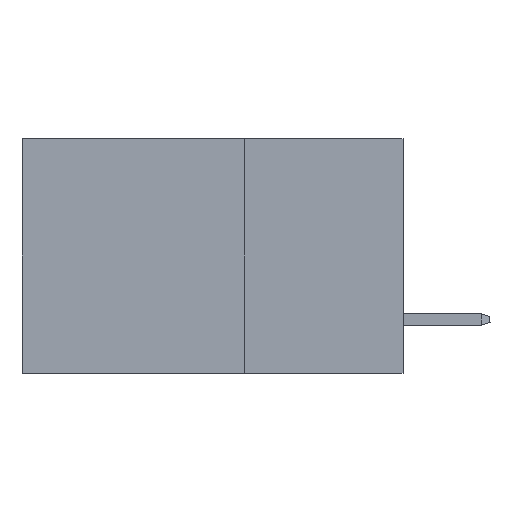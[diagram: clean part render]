
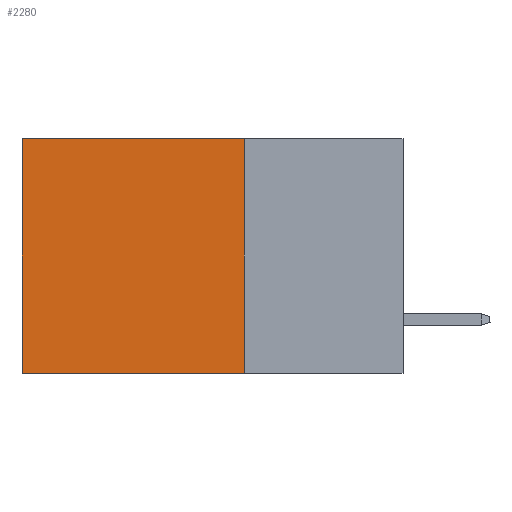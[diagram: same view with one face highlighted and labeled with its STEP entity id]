
A CAD part, left-side view. The second image highlights one B-rep face of the part: STEP entity #2280.
In plain terms, the highlighted planar face has unit normal (-1, 0, 0).
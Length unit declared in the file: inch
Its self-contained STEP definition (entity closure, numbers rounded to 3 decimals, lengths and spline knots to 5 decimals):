
#741 = DIRECTION ( 'NONE',  ( 0., 1., 0. ) ) ;
#2280 = ADVANCED_FACE ( 'NONE', ( #16946 ), #36028, .F. ) ;
#3709 = VERTEX_POINT ( 'NONE', #31649 ) ;
#3940 = CARTESIAN_POINT ( 'NONE',  ( 0.2875, 0.25, -0.37 ) ) ;
#5794 = DIRECTION ( 'NONE',  ( 0., 0., -1. ) ) ;
#5872 = VERTEX_POINT ( 'NONE', #22339 ) ;
#6982 = VECTOR ( 'NONE', #38408, 39.37008 ) ;
#7769 = EDGE_LOOP ( 'NONE', ( #12357, #38991, #22564, #38543 ) ) ;
#12357 = ORIENTED_EDGE ( 'NONE', *, *, #30941, .T. ) ;
#12828 = CARTESIAN_POINT ( 'NONE',  ( 0.2875, 0.25, 0. ) ) ;
#13754 = CARTESIAN_POINT ( 'NONE',  ( 0.2875, 0.25, 0. ) ) ;
#16378 = LINE ( 'NONE', #13754, #24558 ) ;
#16752 = DIRECTION ( 'NONE',  ( 0., 0., -1. ) ) ;
#16913 = CARTESIAN_POINT ( 'NONE',  ( 0.2875, 0.25, -0.37 ) ) ;
#16946 = FACE_OUTER_BOUND ( 'NONE', #7769, .T. ) ;
#17215 = LINE ( 'NONE', #21027, #21004 ) ;
#17308 = VERTEX_POINT ( 'NONE', #29050 ) ;
#17552 = DIRECTION ( 'NONE',  ( 1., 0., 0. ) ) ;
#17915 = LINE ( 'NONE', #12828, #22329 ) ;
#20563 = CARTESIAN_POINT ( 'NONE',  ( 0.2875, 0.25, 0. ) ) ;
#21004 = VECTOR ( 'NONE', #5794, 39.37008 ) ;
#21027 = CARTESIAN_POINT ( 'NONE',  ( 0.2875, 0.6, 0. ) ) ;
#22329 = VECTOR ( 'NONE', #39396, 39.37008 ) ;
#22339 = CARTESIAN_POINT ( 'NONE',  ( 0.2875, 0.25, 0. ) ) ;
#22564 = ORIENTED_EDGE ( 'NONE', *, *, #37671, .F. ) ;
#24558 = VECTOR ( 'NONE', #741, 39.37008 ) ;
#25735 = EDGE_CURVE ( 'NONE', #5872, #17308, #16378, .T. ) ;
#26141 = LINE ( 'NONE', #16913, #6982 ) ;
#29050 = CARTESIAN_POINT ( 'NONE',  ( 0.2875, 0.6, 0. ) ) ;
#29812 = AXIS2_PLACEMENT_3D ( 'NONE', #20563, #17552, #16752 ) ;
#30941 = EDGE_CURVE ( 'NONE', #17308, #3709, #17215, .T. ) ;
#31649 = CARTESIAN_POINT ( 'NONE',  ( 0.2875, 0.6, -0.37 ) ) ;
#33282 = VERTEX_POINT ( 'NONE', #3940 ) ;
#36028 = PLANE ( 'NONE',  #29812 ) ;
#37617 = EDGE_CURVE ( 'NONE', #33282, #3709, #26141, .T. ) ;
#37671 = EDGE_CURVE ( 'NONE', #5872, #33282, #17915, .T. ) ;
#38408 = DIRECTION ( 'NONE',  ( 0., 1., 0. ) ) ;
#38543 = ORIENTED_EDGE ( 'NONE', *, *, #25735, .T. ) ;
#38991 = ORIENTED_EDGE ( 'NONE', *, *, #37617, .F. ) ;
#39396 = DIRECTION ( 'NONE',  ( 0., 0., -1. ) ) ;
